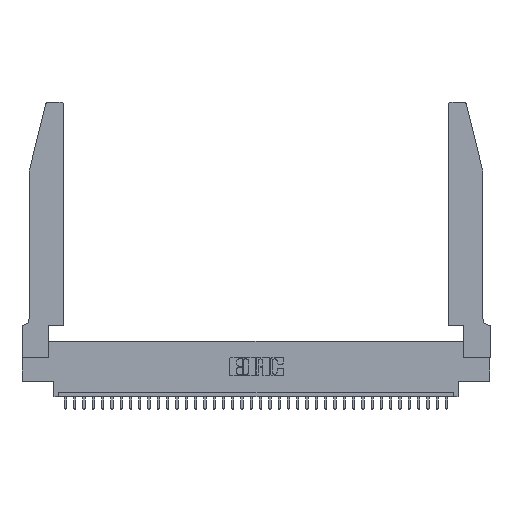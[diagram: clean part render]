
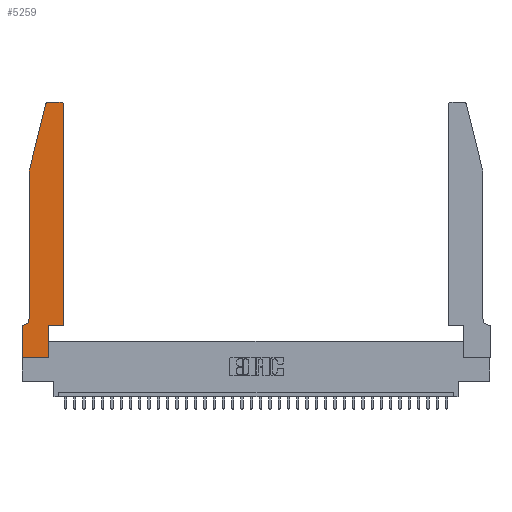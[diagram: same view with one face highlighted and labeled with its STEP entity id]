
A CAD part, top view. The second image highlights one B-rep face of the part: STEP entity #5259.
In plain terms, the highlighted planar face has unit normal (0, 0, 1).
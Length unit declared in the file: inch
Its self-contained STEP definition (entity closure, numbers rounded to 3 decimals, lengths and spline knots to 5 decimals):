
#605 = CARTESIAN_POINT ( 'NONE',  ( 0., 0., 0.37 ) ) ;
#1429 = VECTOR ( 'NONE', #18966, 39.37008 ) ;
#1640 = VERTEX_POINT ( 'NONE', #11025 ) ;
#2062 = CARTESIAN_POINT ( 'NONE',  ( 0., 0., 0.37 ) ) ;
#2079 = LINE ( 'NONE', #2667, #17484 ) ;
#2203 = VERTEX_POINT ( 'NONE', #26266 ) ;
#2667 = CARTESIAN_POINT ( 'NONE',  ( 0.2865, 0.35, 0.37 ) ) ;
#3170 = LINE ( 'NONE', #4798, #1429 ) ;
#3218 = LINE ( 'NONE', #10283, #18667 ) ;
#4096 = ORIENTED_EDGE ( 'NONE', *, *, #23444, .T. ) ;
#4166 = CARTESIAN_POINT ( 'NONE',  ( 0.4205, 2.75, 0.37 ) ) ;
#4784 = CARTESIAN_POINT ( 'NONE',  ( 0.284, 2.75, 0.37 ) ) ;
#4798 = CARTESIAN_POINT ( 'NONE',  ( 0.0755, 2., 0.37 ) ) ;
#5137 = DIRECTION ( 'NONE',  ( 1., 0., 0. ) ) ;
#5193 = CIRCLE ( 'NONE', #14028, 0.03 ) ;
#5259 = ADVANCED_FACE ( 'NONE', ( #27660 ), #19156, .T. ) ;
#6326 = EDGE_CURVE ( 'NONE', #13318, #30769, #5193, .T. ) ;
#9069 = DIRECTION ( 'NONE',  ( 0., -1., 0. ) ) ;
#9485 = VECTOR ( 'NONE', #9069, 39.37008 ) ;
#9517 = CARTESIAN_POINT ( 'NONE',  ( 0.0755, 2., 0.37 ) ) ;
#9624 = CIRCLE ( 'NONE', #31979, 0.03 ) ;
#9937 = ORIENTED_EDGE ( 'NONE', *, *, #12824, .T. ) ;
#10283 = CARTESIAN_POINT ( 'NONE',  ( 0.4505, 0.35, 0.37 ) ) ;
#10905 = ORIENTED_EDGE ( 'NONE', *, *, #16396, .T. ) ;
#11025 = CARTESIAN_POINT ( 'NONE',  ( 0.2865, 0.35, 0.37 ) ) ;
#11338 = VERTEX_POINT ( 'NONE', #29487 ) ;
#12484 = VERTEX_POINT ( 'NONE', #9517 ) ;
#12824 = EDGE_CURVE ( 'NONE', #22857, #2203, #14722, .T. ) ;
#13066 = ORIENTED_EDGE ( 'NONE', *, *, #14885, .T. ) ;
#13074 = ORIENTED_EDGE ( 'NONE', *, *, #30089, .T. ) ;
#13318 = VERTEX_POINT ( 'NONE', #4784 ) ;
#13921 = LINE ( 'NONE', #605, #9485 ) ;
#14028 = AXIS2_PLACEMENT_3D ( 'NONE', #19155, #21736, #21856 ) ;
#14107 = CARTESIAN_POINT ( 'NONE',  ( 0., 0.35, 0.37 ) ) ;
#14431 = VERTEX_POINT ( 'NONE', #30097 ) ;
#14722 = LINE ( 'NONE', #2062, #20449 ) ;
#14885 = EDGE_CURVE ( 'NONE', #11338, #26970, #30287, .T. ) ;
#15649 = EDGE_CURVE ( 'NONE', #2203, #1640, #2079, .T. ) ;
#15672 = CARTESIAN_POINT ( 'NONE',  ( 0., 0.35, 0.37 ) ) ;
#16248 = DIRECTION ( 'NONE',  ( 1., 0., 0. ) ) ;
#16396 = EDGE_CURVE ( 'NONE', #26970, #22857, #13921, .T. ) ;
#16632 = DIRECTION ( 'NONE',  ( 0., 0., 1. ) ) ;
#17417 = DIRECTION ( 'NONE',  ( -1., 0., 0. ) ) ;
#17484 = VECTOR ( 'NONE', #22388, 39.37008 ) ;
#18088 = VECTOR ( 'NONE', #28502, 39.37008 ) ;
#18330 = CARTESIAN_POINT ( 'NONE',  ( 0.25487, 2.72718, 0.37 ) ) ;
#18479 = LINE ( 'NONE', #33281, #27671 ) ;
#18667 = VECTOR ( 'NONE', #5137, 39.37008 ) ;
#18672 = CARTESIAN_POINT ( 'NONE',  ( 0.0755, 0.42, 0.37 ) ) ;
#18966 = DIRECTION ( 'NONE',  ( 0., -1., 0. ) ) ;
#19155 = CARTESIAN_POINT ( 'NONE',  ( 0.284, 2.72, 0.37 ) ) ;
#19156 = PLANE ( 'NONE',  #24359 ) ;
#19773 = AXIS2_PLACEMENT_3D ( 'NONE', #34445, #31814, #29234 ) ;
#20017 = ORIENTED_EDGE ( 'NONE', *, *, #26743, .T. ) ;
#20020 = LINE ( 'NONE', #25798, #26610 ) ;
#20218 = EDGE_CURVE ( 'NONE', #24511, #13318, #20020, .T. ) ;
#20408 = VERTEX_POINT ( 'NONE', #26036 ) ;
#20445 = DIRECTION ( 'NONE',  ( 1., 0., 0. ) ) ;
#20449 = VECTOR ( 'NONE', #16248, 39.37008 ) ;
#20481 = ORIENTED_EDGE ( 'NONE', *, *, #22835, .T. ) ;
#20981 = EDGE_LOOP ( 'NONE', ( #29615, #31236, #20481, #23835, #4096, #13066, #10905, #9937, #31291, #20017, #13074, #24325 ) ) ;
#21435 = EDGE_CURVE ( 'NONE', #12484, #33594, #3170, .T. ) ;
#21736 = DIRECTION ( 'NONE',  ( 0., 0., 1. ) ) ;
#21808 = DIRECTION ( 'NONE',  ( 0., 1., 0. ) ) ;
#21856 = DIRECTION ( 'NONE',  ( 1., 0., 0. ) ) ;
#21941 = CARTESIAN_POINT ( 'NONE',  ( 0.4205, 2.72, 0.37 ) ) ;
#22021 = CIRCLE ( 'NONE', #19773, 0.07 ) ;
#22388 = DIRECTION ( 'NONE',  ( 0., 1., 0. ) ) ;
#22835 = EDGE_CURVE ( 'NONE', #30769, #12484, #25131, .T. ) ;
#22857 = VERTEX_POINT ( 'NONE', #25933 ) ;
#23444 = EDGE_CURVE ( 'NONE', #33594, #11338, #22021, .T. ) ;
#23835 = ORIENTED_EDGE ( 'NONE', *, *, #21435, .T. ) ;
#24067 = CARTESIAN_POINT ( 'NONE',  ( 0.0755, 0.35, 0.37 ) ) ;
#24325 = ORIENTED_EDGE ( 'NONE', *, *, #34377, .T. ) ;
#24359 = AXIS2_PLACEMENT_3D ( 'NONE', #15672, #27469, #20445 ) ;
#24511 = VERTEX_POINT ( 'NONE', #4166 ) ;
#24871 = DIRECTION ( 'NONE',  ( 1., 0., 0. ) ) ;
#25131 = LINE ( 'NONE', #25568, #18088 ) ;
#25568 = CARTESIAN_POINT ( 'NONE',  ( 0.0755, 2., 0.37 ) ) ;
#25798 = CARTESIAN_POINT ( 'NONE',  ( 0.2605, 2.75, 0.37 ) ) ;
#25933 = CARTESIAN_POINT ( 'NONE',  ( 0., 0., 0.37 ) ) ;
#26036 = CARTESIAN_POINT ( 'NONE',  ( 0.4505, 2.72, 0.37 ) ) ;
#26266 = CARTESIAN_POINT ( 'NONE',  ( 0.2865, 0., 0.37 ) ) ;
#26610 = VECTOR ( 'NONE', #17417, 39.37008 ) ;
#26743 = EDGE_CURVE ( 'NONE', #1640, #14431, #3218, .T. ) ;
#26970 = VERTEX_POINT ( 'NONE', #14107 ) ;
#27469 = DIRECTION ( 'NONE',  ( 0., 0., 1. ) ) ;
#27660 = FACE_OUTER_BOUND ( 'NONE', #20981, .T. ) ;
#27671 = VECTOR ( 'NONE', #21808, 39.37008 ) ;
#28502 = DIRECTION ( 'NONE',  ( -0.239, -0.971, 0. ) ) ;
#29234 = DIRECTION ( 'NONE',  ( -1., 0., 0. ) ) ;
#29487 = CARTESIAN_POINT ( 'NONE',  ( 0.0055, 0.35, 0.37 ) ) ;
#29615 = ORIENTED_EDGE ( 'NONE', *, *, #20218, .T. ) ;
#30089 = EDGE_CURVE ( 'NONE', #14431, #20408, #18479, .T. ) ;
#30097 = CARTESIAN_POINT ( 'NONE',  ( 0.4505, 0.35, 0.37 ) ) ;
#30245 = VECTOR ( 'NONE', #35553, 39.37008 ) ;
#30287 = LINE ( 'NONE', #24067, #30245 ) ;
#30769 = VERTEX_POINT ( 'NONE', #18330 ) ;
#31236 = ORIENTED_EDGE ( 'NONE', *, *, #6326, .T. ) ;
#31291 = ORIENTED_EDGE ( 'NONE', *, *, #15649, .T. ) ;
#31814 = DIRECTION ( 'NONE',  ( 0., 0., -1. ) ) ;
#31979 = AXIS2_PLACEMENT_3D ( 'NONE', #21941, #16632, #24871 ) ;
#33281 = CARTESIAN_POINT ( 'NONE',  ( 0.4505, 0.35, 0.37 ) ) ;
#33594 = VERTEX_POINT ( 'NONE', #18672 ) ;
#34377 = EDGE_CURVE ( 'NONE', #20408, #24511, #9624, .T. ) ;
#34445 = CARTESIAN_POINT ( 'NONE',  ( 0.0055, 0.42, 0.37 ) ) ;
#35553 = DIRECTION ( 'NONE',  ( -1., 0., 0. ) ) ;
